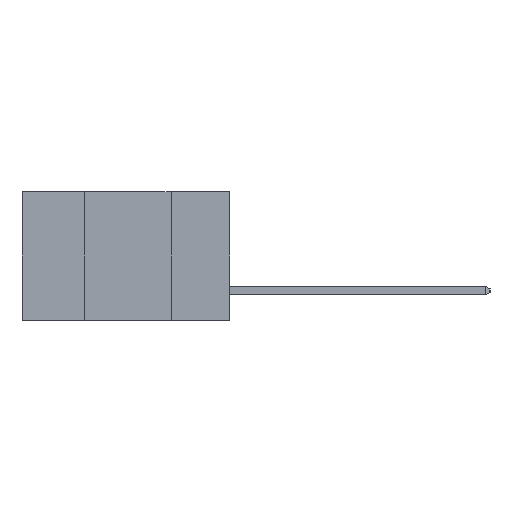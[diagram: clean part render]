
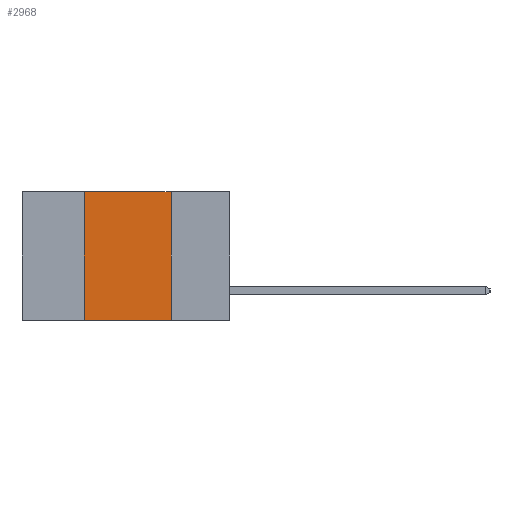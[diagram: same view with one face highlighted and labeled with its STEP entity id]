
A CAD part, left-side view. The second image highlights one B-rep face of the part: STEP entity #2968.
In plain terms, the highlighted planar face has unit normal (-1, 0, 0).
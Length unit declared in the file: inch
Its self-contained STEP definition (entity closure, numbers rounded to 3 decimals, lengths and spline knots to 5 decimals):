
#21 = CARTESIAN_POINT ( 'NONE',  ( 0., 0.17, 0. ) ) ;
#689 = DIRECTION ( 'NONE',  ( 0., 0., -1. ) ) ;
#743 = FACE_OUTER_BOUND ( 'NONE', #17979, .T. ) ;
#907 = DIRECTION ( 'NONE',  ( 0., -1., 0. ) ) ;
#1642 = VERTEX_POINT ( 'NONE', #24707 ) ;
#1791 = EDGE_CURVE ( 'NONE', #28147, #17633, #18655, .T. ) ;
#1837 = VECTOR ( 'NONE', #20249, 39.37008 ) ;
#2968 = ADVANCED_FACE ( 'NONE', ( #743 ), #27916, .F. ) ;
#4449 = ORIENTED_EDGE ( 'NONE', *, *, #6277, .F. ) ;
#4471 = LINE ( 'NONE', #7520, #15448 ) ;
#4737 = VECTOR ( 'NONE', #20885, 39.37008 ) ;
#5227 = AXIS2_PLACEMENT_3D ( 'NONE', #26729, #10711, #689 ) ;
#5399 = VECTOR ( 'NONE', #27096, 39.37008 ) ;
#5446 = LINE ( 'NONE', #14425, #4737 ) ;
#5838 = ORIENTED_EDGE ( 'NONE', *, *, #1791, .F. ) ;
#6277 = EDGE_CURVE ( 'NONE', #16486, #1642, #5446, .T. ) ;
#7520 = CARTESIAN_POINT ( 'NONE',  ( 0., 0.6, 0. ) ) ;
#7606 = CARTESIAN_POINT ( 'NONE',  ( 0., 0.6, -0.37 ) ) ;
#8278 = EDGE_CURVE ( 'NONE', #17633, #16486, #4471, .T. ) ;
#10711 = DIRECTION ( 'NONE',  ( 1., 0., 0. ) ) ;
#11041 = ORIENTED_EDGE ( 'NONE', *, *, #8278, .F. ) ;
#12357 = CARTESIAN_POINT ( 'NONE',  ( 0., 0.42, -0.37 ) ) ;
#14425 = CARTESIAN_POINT ( 'NONE',  ( 0., 0.17, 0. ) ) ;
#15448 = VECTOR ( 'NONE', #907, 39.37008 ) ;
#16486 = VERTEX_POINT ( 'NONE', #21 ) ;
#17464 = ORIENTED_EDGE ( 'NONE', *, *, #18811, .T. ) ;
#17633 = VERTEX_POINT ( 'NONE', #27529 ) ;
#17979 = EDGE_LOOP ( 'NONE', ( #4449, #11041, #5838, #17464 ) ) ;
#18655 = LINE ( 'NONE', #20122, #1837 ) ;
#18811 = EDGE_CURVE ( 'NONE', #28147, #1642, #22735, .T. ) ;
#20122 = CARTESIAN_POINT ( 'NONE',  ( 0., 0.42, 0. ) ) ;
#20249 = DIRECTION ( 'NONE',  ( 0., 0., 1. ) ) ;
#20885 = DIRECTION ( 'NONE',  ( 0., 0., -1. ) ) ;
#22735 = LINE ( 'NONE', #7606, #5399 ) ;
#24707 = CARTESIAN_POINT ( 'NONE',  ( 0., 0.17, -0.37 ) ) ;
#26729 = CARTESIAN_POINT ( 'NONE',  ( 0., 0.6, 0. ) ) ;
#27096 = DIRECTION ( 'NONE',  ( 0., -1., 0. ) ) ;
#27529 = CARTESIAN_POINT ( 'NONE',  ( 0., 0.42, 0. ) ) ;
#27916 = PLANE ( 'NONE',  #5227 ) ;
#28147 = VERTEX_POINT ( 'NONE', #12357 ) ;
